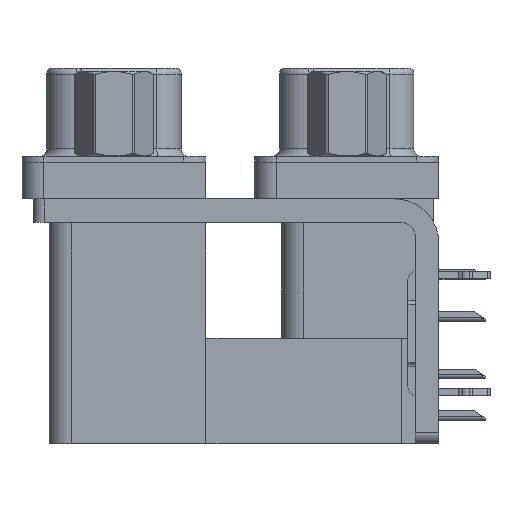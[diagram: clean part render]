
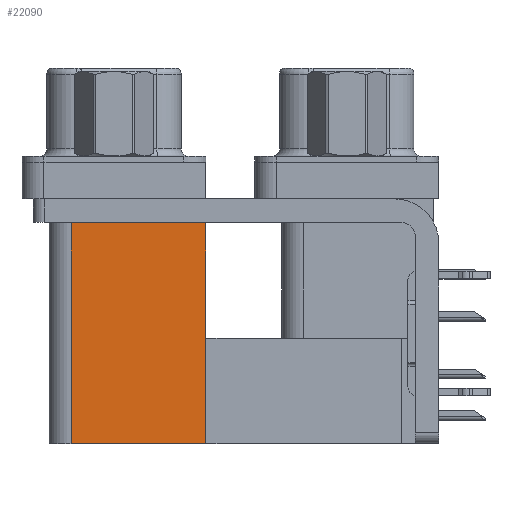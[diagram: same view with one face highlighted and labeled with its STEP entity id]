
A CAD part, left-side view. The second image highlights one B-rep face of the part: STEP entity #22090.
In plain terms, the highlighted planar face has unit normal (-1, 0, 0).
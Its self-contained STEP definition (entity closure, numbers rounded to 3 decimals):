
#3480 = CARTESIAN_POINT ( 'NONE',  ( 3.765, 18.8, -2.5 ) ) ;
#6067 = EDGE_CURVE ( 'NONE', #24706, #16002, #8481, .T. ) ;
#7439 = CARTESIAN_POINT ( 'NONE',  ( 3.765, 9.6, -19.2 ) ) ;
#7579 = AXIS2_PLACEMENT_3D ( 'NONE', #27326, #24177, #11801 ) ;
#8481 = LINE ( 'NONE', #11835, #24695 ) ;
#10259 = LINE ( 'NONE', #18328, #14677 ) ;
#11801 = DIRECTION ( 'NONE',  ( 0., 0., -1. ) ) ;
#11835 = CARTESIAN_POINT ( 'NONE',  ( 3.765, 9.6, -19.2 ) ) ;
#14677 = VECTOR ( 'NONE', #18526, 1000. ) ;
#14775 = EDGE_LOOP ( 'NONE', ( #20465, #15785, #18736, #34777 ) ) ;
#15461 = CARTESIAN_POINT ( 'NONE',  ( 3.765, 18.8, -19.2 ) ) ;
#15785 = ORIENTED_EDGE ( 'NONE', *, *, #33493, .F. ) ;
#15883 = CARTESIAN_POINT ( 'NONE',  ( 3.765, 9.6, -19.2 ) ) ;
#16002 = VERTEX_POINT ( 'NONE', #15461 ) ;
#18328 = CARTESIAN_POINT ( 'NONE',  ( 3.765, 18.8, -19.2 ) ) ;
#18496 = EDGE_CURVE ( 'NONE', #32361, #24597, #24561, .T. ) ;
#18526 = DIRECTION ( 'NONE',  ( 0., 0., 1. ) ) ;
#18736 = ORIENTED_EDGE ( 'NONE', *, *, #6067, .F. ) ;
#19328 = VECTOR ( 'NONE', #34365, 1000. ) ;
#19968 = VECTOR ( 'NONE', #24953, 1000. ) ;
#20465 = ORIENTED_EDGE ( 'NONE', *, *, #18496, .T. ) ;
#22090 = ADVANCED_FACE ( 'NONE', ( #33392 ), #35761, .F. ) ;
#23432 = DIRECTION ( 'NONE',  ( 0., 1., 0. ) ) ;
#24177 = DIRECTION ( 'NONE',  ( 1., 0., 0. ) ) ;
#24561 = LINE ( 'NONE', #37299, #19968 ) ;
#24597 = VERTEX_POINT ( 'NONE', #3480 ) ;
#24695 = VECTOR ( 'NONE', #23432, 1000. ) ;
#24706 = VERTEX_POINT ( 'NONE', #15883 ) ;
#24953 = DIRECTION ( 'NONE',  ( 0., 1., 0. ) ) ;
#27326 = CARTESIAN_POINT ( 'NONE',  ( 3.765, 9.6, -19.2 ) ) ;
#27894 = LINE ( 'NONE', #7439, #19328 ) ;
#32361 = VERTEX_POINT ( 'NONE', #32950 ) ;
#32950 = CARTESIAN_POINT ( 'NONE',  ( 3.765, 9.6, -2.5 ) ) ;
#33392 = FACE_OUTER_BOUND ( 'NONE', #14775, .T. ) ;
#33493 = EDGE_CURVE ( 'NONE', #16002, #24597, #10259, .T. ) ;
#34365 = DIRECTION ( 'NONE',  ( 0., 0., 1. ) ) ;
#34777 = ORIENTED_EDGE ( 'NONE', *, *, #38563, .T. ) ;
#35761 = PLANE ( 'NONE',  #7579 ) ;
#37299 = CARTESIAN_POINT ( 'NONE',  ( 3.765, 9.6, -2.5 ) ) ;
#38563 = EDGE_CURVE ( 'NONE', #24706, #32361, #27894, .T. ) ;
